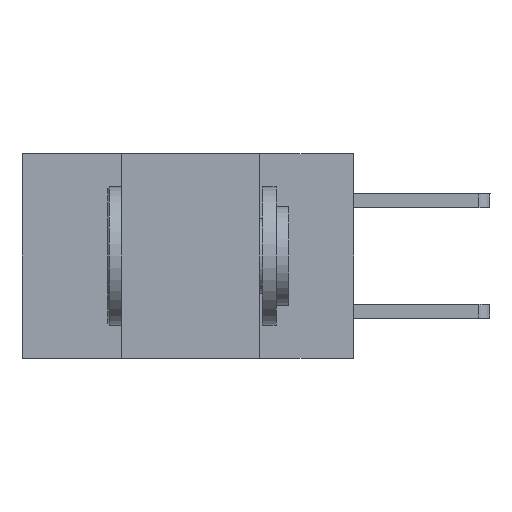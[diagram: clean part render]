
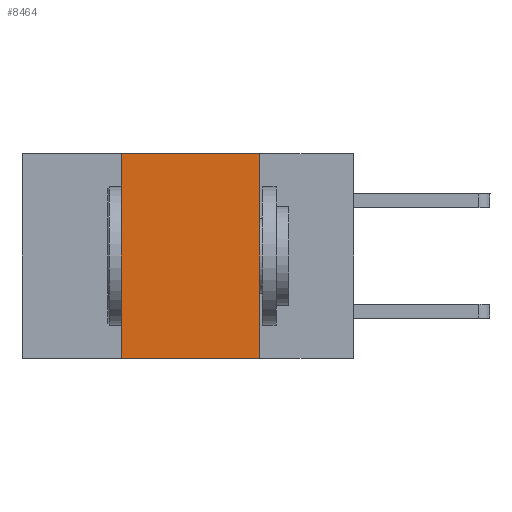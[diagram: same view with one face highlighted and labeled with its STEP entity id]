
A CAD part, left-side view. The second image highlights one B-rep face of the part: STEP entity #8464.
In plain terms, the highlighted planar face has unit normal (-1, 0, 0).
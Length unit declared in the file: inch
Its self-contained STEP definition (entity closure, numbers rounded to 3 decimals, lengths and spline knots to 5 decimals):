
#99 = DIRECTION ( 'NONE',  ( 0., 0., -1. ) ) ;
#309 = AXIS2_PLACEMENT_3D ( 'NONE', #8064, #5586, #9665 ) ;
#498 = CARTESIAN_POINT ( 'NONE',  ( 0., 0.17, -0.37 ) ) ;
#635 = CARTESIAN_POINT ( 'NONE',  ( 0., 0.17, 0. ) ) ;
#1034 = FACE_OUTER_BOUND ( 'NONE', #2210, .T. ) ;
#1865 = VECTOR ( 'NONE', #10744, 39.37008 ) ;
#2156 = VECTOR ( 'NONE', #99, 39.37008 ) ;
#2210 = EDGE_LOOP ( 'NONE', ( #5694, #2638, #6614, #9869 ) ) ;
#2638 = ORIENTED_EDGE ( 'NONE', *, *, #3692, .F. ) ;
#3174 = CARTESIAN_POINT ( 'NONE',  ( 0., 0.17, 0. ) ) ;
#3692 = EDGE_CURVE ( 'NONE', #7237, #10260, #4594, .T. ) ;
#4550 = LINE ( 'NONE', #10903, #8653 ) ;
#4594 = LINE ( 'NONE', #7259, #6450 ) ;
#4619 = CARTESIAN_POINT ( 'NONE',  ( 0., 0.42, 0. ) ) ;
#4709 = EDGE_CURVE ( 'NONE', #10260, #10379, #6975, .T. ) ;
#4711 = EDGE_CURVE ( 'NONE', #5009, #7237, #4550, .T. ) ;
#4725 = EDGE_CURVE ( 'NONE', #5009, #10379, #6408, .T. ) ;
#5009 = VERTEX_POINT ( 'NONE', #7173 ) ;
#5586 = DIRECTION ( 'NONE',  ( 1., 0., 0. ) ) ;
#5694 = ORIENTED_EDGE ( 'NONE', *, *, #4709, .F. ) ;
#6364 = DIRECTION ( 'NONE',  ( 0., -1., 0. ) ) ;
#6408 = LINE ( 'NONE', #10714, #1865 ) ;
#6450 = VECTOR ( 'NONE', #6364, 39.37008 ) ;
#6614 = ORIENTED_EDGE ( 'NONE', *, *, #4711, .F. ) ;
#6975 = LINE ( 'NONE', #635, #2156 ) ;
#7173 = CARTESIAN_POINT ( 'NONE',  ( 0., 0.42, -0.37 ) ) ;
#7237 = VERTEX_POINT ( 'NONE', #4619 ) ;
#7259 = CARTESIAN_POINT ( 'NONE',  ( 0., 0.6, 0. ) ) ;
#8064 = CARTESIAN_POINT ( 'NONE',  ( 0., 0.6, 0. ) ) ;
#8464 = ADVANCED_FACE ( 'NONE', ( #1034 ), #8863, .F. ) ;
#8653 = VECTOR ( 'NONE', #10826, 39.37008 ) ;
#8863 = PLANE ( 'NONE',  #309 ) ;
#9665 = DIRECTION ( 'NONE',  ( 0., 0., -1. ) ) ;
#9869 = ORIENTED_EDGE ( 'NONE', *, *, #4725, .T. ) ;
#10260 = VERTEX_POINT ( 'NONE', #3174 ) ;
#10379 = VERTEX_POINT ( 'NONE', #498 ) ;
#10714 = CARTESIAN_POINT ( 'NONE',  ( 0., 0.6, -0.37 ) ) ;
#10744 = DIRECTION ( 'NONE',  ( 0., -1., 0. ) ) ;
#10826 = DIRECTION ( 'NONE',  ( 0., 0., 1. ) ) ;
#10903 = CARTESIAN_POINT ( 'NONE',  ( 0., 0.42, 0. ) ) ;
